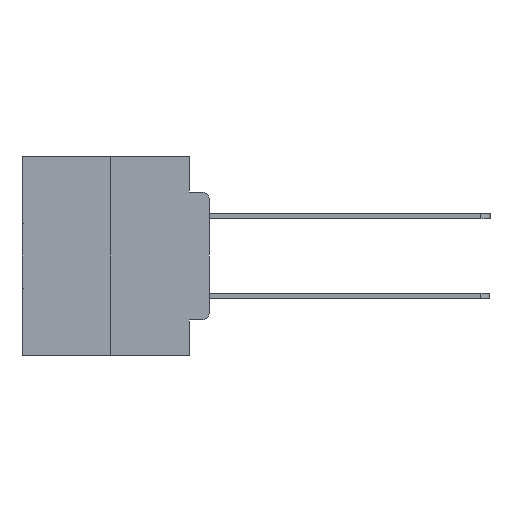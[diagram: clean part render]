
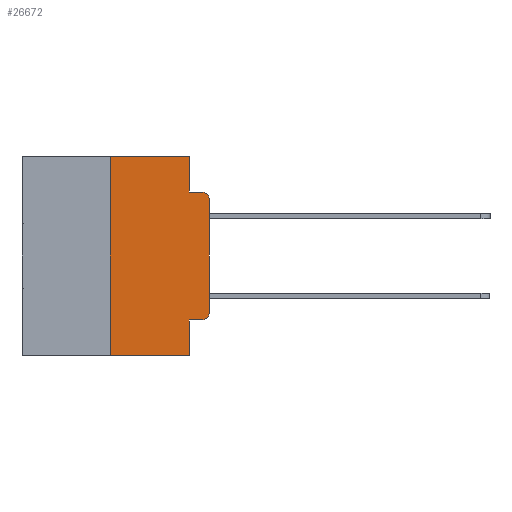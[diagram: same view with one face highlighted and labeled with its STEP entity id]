
A CAD part, left-side view. The second image highlights one B-rep face of the part: STEP entity #26672.
In plain terms, the highlighted planar face has unit normal (-1, 0, 0).
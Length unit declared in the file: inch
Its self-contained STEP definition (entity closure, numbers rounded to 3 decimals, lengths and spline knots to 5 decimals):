
#67 = LINE ( 'NONE', #11222, #22980 ) ;
#632 = CARTESIAN_POINT ( 'NONE',  ( 0., 0., -0.1085 ) ) ;
#641 = VECTOR ( 'NONE', #13671, 39.37008 ) ;
#975 = EDGE_CURVE ( 'NONE', #7215, #3987, #5406, .T. ) ;
#1199 = ORIENTED_EDGE ( 'NONE', *, *, #22113, .T. ) ;
#1539 = ORIENTED_EDGE ( 'NONE', *, *, #15309, .T. ) ;
#1883 = DIRECTION ( 'NONE',  ( 0., 0., -1. ) ) ;
#2107 = LINE ( 'NONE', #18042, #641 ) ;
#2165 = CARTESIAN_POINT ( 'NONE',  ( 0., 0.25, 0. ) ) ;
#3002 = ORIENTED_EDGE ( 'NONE', *, *, #18204, .T. ) ;
#3668 = VECTOR ( 'NONE', #26855, 39.37008 ) ;
#3987 = VERTEX_POINT ( 'NONE', #12540 ) ;
#4414 = DIRECTION ( 'NONE',  ( 0., 0., -1. ) ) ;
#4542 = EDGE_CURVE ( 'NONE', #10852, #7215, #25752, .T. ) ;
#4734 = CARTESIAN_POINT ( 'NONE',  ( 0., 0.25, -0.5 ) ) ;
#5406 = LINE ( 'NONE', #10484, #6130 ) ;
#6062 = EDGE_CURVE ( 'NONE', #27206, #21745, #67, .T. ) ;
#6130 = VECTOR ( 'NONE', #10348, 39.37008 ) ;
#6186 = DIRECTION ( 'NONE',  ( 0., 0., -1. ) ) ;
#6620 = VECTOR ( 'NONE', #6186, 39.37008 ) ;
#7215 = VERTEX_POINT ( 'NONE', #25983 ) ;
#7337 = LINE ( 'NONE', #15001, #6620 ) ;
#8683 = LINE ( 'NONE', #11512, #25319 ) ;
#8869 = CARTESIAN_POINT ( 'NONE',  ( 0., 0.473, 0. ) ) ;
#9286 = AXIS2_PLACEMENT_3D ( 'NONE', #11257, #26356, #13443 ) ;
#9445 = CARTESIAN_POINT ( 'NONE',  ( 0., 0.02, -0.0885 ) ) ;
#9651 = CARTESIAN_POINT ( 'NONE',  ( 0., 0.051, -0.4115 ) ) ;
#9840 = VECTOR ( 'NONE', #21726, 39.37008 ) ;
#10348 = DIRECTION ( 'NONE',  ( 0., -1., 0. ) ) ;
#10461 = ORIENTED_EDGE ( 'NONE', *, *, #17507, .F. ) ;
#10484 = CARTESIAN_POINT ( 'NONE',  ( 0., 0.473, 0. ) ) ;
#10852 = VERTEX_POINT ( 'NONE', #4734 ) ;
#11060 = CARTESIAN_POINT ( 'NONE',  ( 0., 0.02, -0.4115 ) ) ;
#11105 = PLANE ( 'NONE',  #16038 ) ;
#11222 = CARTESIAN_POINT ( 'NONE',  ( 0., 0.051, 0. ) ) ;
#11257 = CARTESIAN_POINT ( 'NONE',  ( 0., 0.02, -0.1085 ) ) ;
#11489 = CIRCLE ( 'NONE', #9286, 0.02 ) ;
#11512 = CARTESIAN_POINT ( 'NONE',  ( 0., 0.473, -0.5 ) ) ;
#11816 = ORIENTED_EDGE ( 'NONE', *, *, #975, .F. ) ;
#11869 = LINE ( 'NONE', #15626, #12541 ) ;
#12526 = VERTEX_POINT ( 'NONE', #9445 ) ;
#12540 = CARTESIAN_POINT ( 'NONE',  ( 0., 0.051, 0. ) ) ;
#12541 = VECTOR ( 'NONE', #19868, 39.37008 ) ;
#12960 = CARTESIAN_POINT ( 'NONE',  ( 0., 0.051, -0.4115 ) ) ;
#13443 = DIRECTION ( 'NONE',  ( 0., 0., -1. ) ) ;
#13508 = EDGE_CURVE ( 'NONE', #23607, #12526, #11869, .T. ) ;
#13671 = DIRECTION ( 'NONE',  ( 0., 0., 1. ) ) ;
#14049 = EDGE_CURVE ( 'NONE', #16340, #25749, #19830, .T. ) ;
#14234 = ORIENTED_EDGE ( 'NONE', *, *, #14049, .T. ) ;
#14323 = CARTESIAN_POINT ( 'NONE',  ( 0., 0., -0.3915 ) ) ;
#15001 = CARTESIAN_POINT ( 'NONE',  ( 0., 0.051, 0. ) ) ;
#15309 = EDGE_CURVE ( 'NONE', #25749, #20979, #2107, .T. ) ;
#15315 = DIRECTION ( 'NONE',  ( -1., 0., 0. ) ) ;
#15609 = DIRECTION ( 'NONE',  ( 0., 0., -1. ) ) ;
#15626 = CARTESIAN_POINT ( 'NONE',  ( 0., 0.051, -0.0885 ) ) ;
#16038 = AXIS2_PLACEMENT_3D ( 'NONE', #8869, #17664, #4414 ) ;
#16191 = EDGE_LOOP ( 'NONE', ( #1539, #3002, #19273, #10461, #11816, #28284, #1199, #24004, #18952, #14234 ) ) ;
#16340 = VERTEX_POINT ( 'NONE', #11060 ) ;
#17507 = EDGE_CURVE ( 'NONE', #3987, #23607, #7337, .T. ) ;
#17664 = DIRECTION ( 'NONE',  ( 1., 0., 0. ) ) ;
#18042 = CARTESIAN_POINT ( 'NONE',  ( 0., 0., 0. ) ) ;
#18204 = EDGE_CURVE ( 'NONE', #20979, #12526, #11489, .T. ) ;
#18738 = FACE_OUTER_BOUND ( 'NONE', #16191, .T. ) ;
#18952 = ORIENTED_EDGE ( 'NONE', *, *, #22723, .T. ) ;
#19273 = ORIENTED_EDGE ( 'NONE', *, *, #13508, .F. ) ;
#19830 = CIRCLE ( 'NONE', #23231, 0.02 ) ;
#19868 = DIRECTION ( 'NONE',  ( 0., -1., 0. ) ) ;
#20568 = LINE ( 'NONE', #9651, #3668 ) ;
#20979 = VERTEX_POINT ( 'NONE', #632 ) ;
#21726 = DIRECTION ( 'NONE',  ( 0., 0., 1. ) ) ;
#21745 = VERTEX_POINT ( 'NONE', #25329 ) ;
#22113 = EDGE_CURVE ( 'NONE', #10852, #21745, #8683, .T. ) ;
#22723 = EDGE_CURVE ( 'NONE', #27206, #16340, #20568, .T. ) ;
#22980 = VECTOR ( 'NONE', #15609, 39.37008 ) ;
#23231 = AXIS2_PLACEMENT_3D ( 'NONE', #28115, #15315, #1883 ) ;
#23607 = VERTEX_POINT ( 'NONE', #26203 ) ;
#24004 = ORIENTED_EDGE ( 'NONE', *, *, #6062, .F. ) ;
#25319 = VECTOR ( 'NONE', #26614, 39.37008 ) ;
#25329 = CARTESIAN_POINT ( 'NONE',  ( 0., 0.051, -0.5 ) ) ;
#25749 = VERTEX_POINT ( 'NONE', #14323 ) ;
#25752 = LINE ( 'NONE', #2165, #9840 ) ;
#25983 = CARTESIAN_POINT ( 'NONE',  ( 0., 0.25, 0. ) ) ;
#26203 = CARTESIAN_POINT ( 'NONE',  ( 0., 0.051, -0.0885 ) ) ;
#26356 = DIRECTION ( 'NONE',  ( -1., 0., 0. ) ) ;
#26614 = DIRECTION ( 'NONE',  ( 0., -1., 0. ) ) ;
#26672 = ADVANCED_FACE ( 'NONE', ( #18738 ), #11105, .F. ) ;
#26855 = DIRECTION ( 'NONE',  ( 0., -1., 0. ) ) ;
#27206 = VERTEX_POINT ( 'NONE', #12960 ) ;
#28115 = CARTESIAN_POINT ( 'NONE',  ( 0., 0.02, -0.3915 ) ) ;
#28284 = ORIENTED_EDGE ( 'NONE', *, *, #4542, .F. ) ;
